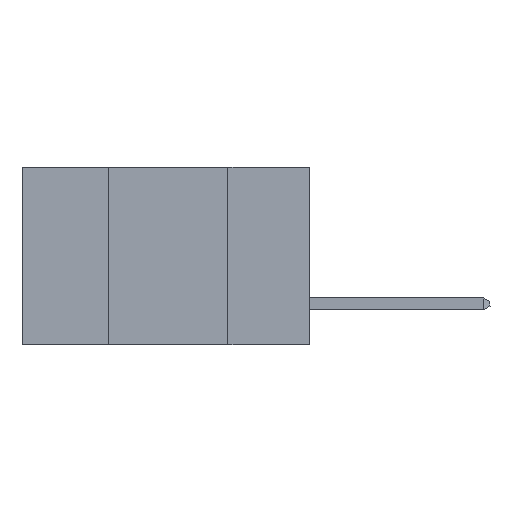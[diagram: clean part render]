
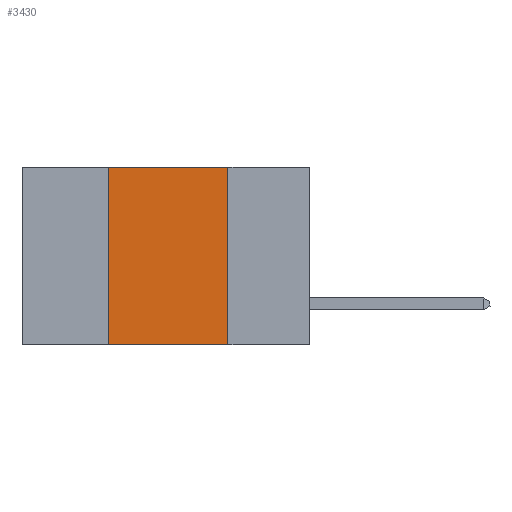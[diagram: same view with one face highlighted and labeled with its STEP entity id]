
A CAD part, left-side view. The second image highlights one B-rep face of the part: STEP entity #3430.
In plain terms, the highlighted planar face has unit normal (-1, 0, 0).
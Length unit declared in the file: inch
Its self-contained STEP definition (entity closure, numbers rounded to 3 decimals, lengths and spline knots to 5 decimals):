
#135 = VERTEX_POINT ( 'NONE', #6717 ) ;
#167 = VECTOR ( 'NONE', #9878, 39.37008 ) ;
#282 = EDGE_CURVE ( 'NONE', #135, #2049, #9747, .T. ) ;
#370 = EDGE_CURVE ( 'NONE', #2049, #7574, #9304, .T. ) ;
#450 = CARTESIAN_POINT ( 'NONE',  ( 0., 0.17, 0. ) ) ;
#475 = LINE ( 'NONE', #3390, #167 ) ;
#1059 = EDGE_CURVE ( 'NONE', #9552, #135, #475, .T. ) ;
#1164 = CARTESIAN_POINT ( 'NONE',  ( 0., 0.6, -0.37 ) ) ;
#1268 = VECTOR ( 'NONE', #8566, 39.37008 ) ;
#1660 = FACE_OUTER_BOUND ( 'NONE', #8991, .T. ) ;
#1688 = EDGE_CURVE ( 'NONE', #9552, #7574, #4057, .T. ) ;
#1758 = CARTESIAN_POINT ( 'NONE',  ( 0., 0.42, -0.37 ) ) ;
#1930 = DIRECTION ( 'NONE',  ( 0., 0., -1. ) ) ;
#1970 = ORIENTED_EDGE ( 'NONE', *, *, #1688, .T. ) ;
#2049 = VERTEX_POINT ( 'NONE', #450 ) ;
#3081 = DIRECTION ( 'NONE',  ( 0., -1., 0. ) ) ;
#3390 = CARTESIAN_POINT ( 'NONE',  ( 0., 0.42, 0. ) ) ;
#3430 = ADVANCED_FACE ( 'NONE', ( #1660 ), #9891, .F. ) ;
#4057 = LINE ( 'NONE', #1164, #6065 ) ;
#4976 = ORIENTED_EDGE ( 'NONE', *, *, #282, .F. ) ;
#4983 = VECTOR ( 'NONE', #1930, 39.37008 ) ;
#5503 = DIRECTION ( 'NONE',  ( 1., 0., 0. ) ) ;
#5896 = CARTESIAN_POINT ( 'NONE',  ( 0., 0.6, 0. ) ) ;
#5976 = CARTESIAN_POINT ( 'NONE',  ( 0., 0.17, 0. ) ) ;
#6065 = VECTOR ( 'NONE', #3081, 39.37008 ) ;
#6717 = CARTESIAN_POINT ( 'NONE',  ( 0., 0.42, 0. ) ) ;
#7572 = ORIENTED_EDGE ( 'NONE', *, *, #1059, .F. ) ;
#7574 = VERTEX_POINT ( 'NONE', #8576 ) ;
#7747 = ORIENTED_EDGE ( 'NONE', *, *, #370, .F. ) ;
#7804 = AXIS2_PLACEMENT_3D ( 'NONE', #5896, #5503, #8635 ) ;
#8566 = DIRECTION ( 'NONE',  ( 0., -1., 0. ) ) ;
#8576 = CARTESIAN_POINT ( 'NONE',  ( 0., 0.17, -0.37 ) ) ;
#8628 = CARTESIAN_POINT ( 'NONE',  ( 0., 0.6, 0. ) ) ;
#8635 = DIRECTION ( 'NONE',  ( 0., 0., -1. ) ) ;
#8991 = EDGE_LOOP ( 'NONE', ( #7747, #4976, #7572, #1970 ) ) ;
#9304 = LINE ( 'NONE', #5976, #4983 ) ;
#9552 = VERTEX_POINT ( 'NONE', #1758 ) ;
#9747 = LINE ( 'NONE', #8628, #1268 ) ;
#9878 = DIRECTION ( 'NONE',  ( 0., 0., 1. ) ) ;
#9891 = PLANE ( 'NONE',  #7804 ) ;
